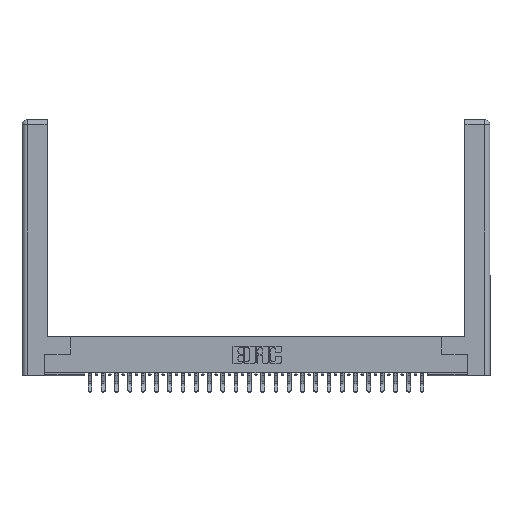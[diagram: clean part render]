
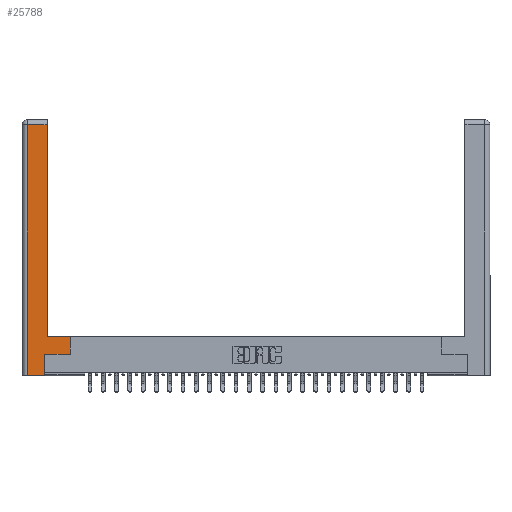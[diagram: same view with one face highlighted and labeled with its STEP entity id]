
A CAD part, top view. The second image highlights one B-rep face of the part: STEP entity #25788.
In plain terms, the highlighted planar face has unit normal (0, 0, 1).
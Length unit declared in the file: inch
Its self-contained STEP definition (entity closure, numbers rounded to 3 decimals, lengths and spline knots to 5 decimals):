
#5 = LINE ( 'NONE', #15356, #6382 ) ;
#88 = DIRECTION ( 'NONE',  ( 0., 1., 0. ) ) ;
#1765 = EDGE_LOOP ( 'NONE', ( #28666, #2186, #10747, #7359, #20329, #20473, #30891, #9760 ) ) ;
#1908 = CARTESIAN_POINT ( 'NONE',  ( 0.295, 0.45, 0. ) ) ;
#2186 = ORIENTED_EDGE ( 'NONE', *, *, #16267, .T. ) ;
#2263 = CARTESIAN_POINT ( 'NONE',  ( 0.265, 0., 0. ) ) ;
#2730 = VECTOR ( 'NONE', #25770, 39.37008 ) ;
#2971 = CARTESIAN_POINT ( 'NONE',  ( 0.0615, 2.94, 0. ) ) ;
#3033 = EDGE_CURVE ( 'NONE', #25447, #22269, #25342, .T. ) ;
#3309 = DIRECTION ( 'NONE',  ( 1., 0., 0. ) ) ;
#5059 = EDGE_CURVE ( 'NONE', #14258, #9658, #5, .T. ) ;
#5813 = CARTESIAN_POINT ( 'NONE',  ( 0.0615, 0., 0. ) ) ;
#6012 = CARTESIAN_POINT ( 'NONE',  ( 0.265, 0.245, 0. ) ) ;
#6382 = VECTOR ( 'NONE', #88, 39.37008 ) ;
#6468 = DIRECTION ( 'NONE',  ( 0., 1., 0. ) ) ;
#7359 = ORIENTED_EDGE ( 'NONE', *, *, #14000, .T. ) ;
#8226 = DIRECTION ( 'NONE',  ( -1., 0., 0. ) ) ;
#8545 = EDGE_CURVE ( 'NONE', #15191, #23189, #27624, .T. ) ;
#8855 = VERTEX_POINT ( 'NONE', #30797 ) ;
#8966 = CARTESIAN_POINT ( 'NONE',  ( 0., 0., 0. ) ) ;
#9658 = VERTEX_POINT ( 'NONE', #21130 ) ;
#9760 = ORIENTED_EDGE ( 'NONE', *, *, #10770, .T. ) ;
#9856 = DIRECTION ( 'NONE',  ( 0., 1., 0. ) ) ;
#9930 = LINE ( 'NONE', #25551, #2730 ) ;
#10747 = ORIENTED_EDGE ( 'NONE', *, *, #3033, .T. ) ;
#10770 = EDGE_CURVE ( 'NONE', #13378, #14258, #14989, .T. ) ;
#11190 = LINE ( 'NONE', #12609, #16370 ) ;
#12609 = CARTESIAN_POINT ( 'NONE',  ( 0.565, 0.45, 0. ) ) ;
#13378 = VERTEX_POINT ( 'NONE', #27892 ) ;
#13718 = CARTESIAN_POINT ( 'NONE',  ( 0.265, 0.245, 0. ) ) ;
#14000 = EDGE_CURVE ( 'NONE', #22269, #15191, #28640, .T. ) ;
#14034 = DIRECTION ( 'NONE',  ( 0., -1., 0. ) ) ;
#14258 = VERTEX_POINT ( 'NONE', #1908 ) ;
#14393 = DIRECTION ( 'NONE',  ( 0., 0., -1. ) ) ;
#14989 = LINE ( 'NONE', #28643, #20937 ) ;
#15191 = VERTEX_POINT ( 'NONE', #2263 ) ;
#15356 = CARTESIAN_POINT ( 'NONE',  ( 0.295, 3., 0. ) ) ;
#15757 = DIRECTION ( 'NONE',  ( -1., 0., 0. ) ) ;
#15794 = LINE ( 'NONE', #2971, #28522 ) ;
#16267 = EDGE_CURVE ( 'NONE', #9658, #25447, #15794, .T. ) ;
#16370 = VECTOR ( 'NONE', #9856, 39.37008 ) ;
#18475 = EDGE_CURVE ( 'NONE', #23189, #8855, #9930, .T. ) ;
#20329 = ORIENTED_EDGE ( 'NONE', *, *, #8545, .T. ) ;
#20473 = ORIENTED_EDGE ( 'NONE', *, *, #18475, .T. ) ;
#20937 = VECTOR ( 'NONE', #15757, 39.37008 ) ;
#21130 = CARTESIAN_POINT ( 'NONE',  ( 0.295, 2.94, 0. ) ) ;
#21598 = CARTESIAN_POINT ( 'NONE',  ( 0.0615, 0., 0. ) ) ;
#22098 = FACE_OUTER_BOUND ( 'NONE', #1765, .T. ) ;
#22130 = AXIS2_PLACEMENT_3D ( 'NONE', #8966, #14393, #26900 ) ;
#22145 = VECTOR ( 'NONE', #14034, 39.37008 ) ;
#22269 = VERTEX_POINT ( 'NONE', #5813 ) ;
#23189 = VERTEX_POINT ( 'NONE', #6012 ) ;
#25342 = LINE ( 'NONE', #21598, #22145 ) ;
#25447 = VERTEX_POINT ( 'NONE', #27940 ) ;
#25551 = CARTESIAN_POINT ( 'NONE',  ( 0.565, 0.245, 0. ) ) ;
#25770 = DIRECTION ( 'NONE',  ( 1., 0., 0. ) ) ;
#25788 = ADVANCED_FACE ( 'NONE', ( #22098 ), #29606, .F. ) ;
#26162 = CARTESIAN_POINT ( 'NONE',  ( 0.265, 0., 0. ) ) ;
#26900 = DIRECTION ( 'NONE',  ( -1., 0., 0. ) ) ;
#27624 = LINE ( 'NONE', #13718, #29936 ) ;
#27727 = EDGE_CURVE ( 'NONE', #8855, #13378, #11190, .T. ) ;
#27892 = CARTESIAN_POINT ( 'NONE',  ( 0.565, 0.45, 0. ) ) ;
#27940 = CARTESIAN_POINT ( 'NONE',  ( 0.0615, 2.94, 0. ) ) ;
#28522 = VECTOR ( 'NONE', #8226, 39.37008 ) ;
#28640 = LINE ( 'NONE', #26162, #29430 ) ;
#28643 = CARTESIAN_POINT ( 'NONE',  ( 0.295, 0.45, 0. ) ) ;
#28666 = ORIENTED_EDGE ( 'NONE', *, *, #5059, .T. ) ;
#29430 = VECTOR ( 'NONE', #3309, 39.37008 ) ;
#29606 = PLANE ( 'NONE',  #22130 ) ;
#29936 = VECTOR ( 'NONE', #6468, 39.37008 ) ;
#30797 = CARTESIAN_POINT ( 'NONE',  ( 0.565, 0.245, 0. ) ) ;
#30891 = ORIENTED_EDGE ( 'NONE', *, *, #27727, .T. ) ;
